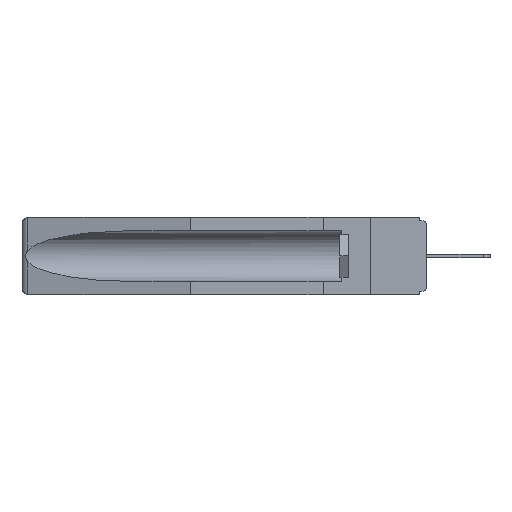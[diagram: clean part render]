
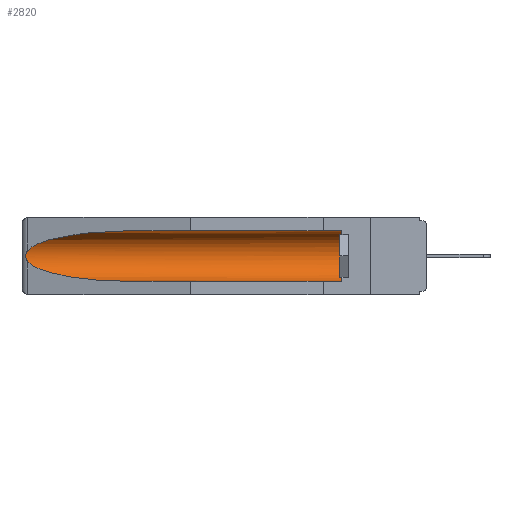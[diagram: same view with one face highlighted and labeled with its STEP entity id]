
A CAD part, left-side view. The second image highlights one B-rep face of the part: STEP entity #2820.
In plain terms, the highlighted cylindrical face has radius 2.857 mm (diameter 5.715 mm), a partial arc.
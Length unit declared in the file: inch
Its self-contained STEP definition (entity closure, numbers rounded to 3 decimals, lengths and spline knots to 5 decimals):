
#394 = VECTOR ( 'NONE', #4092, 39.37008 ) ;
#422 = EDGE_CURVE ( 'NONE', #11254, #11339, #4808, .T. ) ;
#930 = LINE ( 'NONE', #2352, #394 ) ;
#1108 = DIRECTION ( 'NONE',  ( 0., -1., 0. ) ) ;
#1222 = CARTESIAN_POINT ( 'NONE',  ( 0.26654, 1.53092, -0.15636 ) ) ;
#2047 = CARTESIAN_POINT ( 'NONE',  ( 0.155, 1.07973, -0.059 ) ) ;
#2258 = DIRECTION ( 'NONE',  ( 0., 1., 0. ) ) ;
#2352 = CARTESIAN_POINT ( 'NONE',  ( 0.155, -0.30754, -0.284 ) ) ;
#2424 = CARTESIAN_POINT ( 'NONE',  ( 0.155, -0.30754, -0.059 ) ) ;
#2436 = CARTESIAN_POINT ( 'NONE',  ( 0.155, 1.07973, -0.284 ) ) ;
#2820 = ADVANCED_FACE ( 'NONE', ( #14255 ), #13746, .F. ) ;
#2947 = CARTESIAN_POINT ( 'NONE',  ( 0.2675, 1.53308, -0.16763 ) ) ;
#3113 = CARTESIAN_POINT ( 'NONE',  ( 0.155, 1.07973, -0.059 ) ) ;
#3420 = CARTESIAN_POINT ( 'NONE',  ( 0.25451, 1.48313, -0.24835 ) ) ;
#3496 = CARTESIAN_POINT ( 'NONE',  ( 0.155, 1.07973, -0.284 ) ) ;
#3936 = AXIS2_PLACEMENT_3D ( 'NONE', #11329, #1108, #13002 ) ;
#4009 = ORIENTED_EDGE ( 'NONE', *, *, #20842, .T. ) ;
#4092 = DIRECTION ( 'NONE',  ( 0., 1., 0. ) ) ;
#4659 = CARTESIAN_POINT ( 'NONE',  ( 0.2673, 1.53269, -0.17917 ) ) ;
#4808 = LINE ( 'NONE', #2424, #13302 ) ;
#6297 = CARTESIAN_POINT ( 'NONE',  ( 0.26537, 1.52718, -0.14972 ) ) ;
#6304 = ORIENTED_EDGE ( 'NONE', *, *, #8364, .T. ) ;
#6366 = CARTESIAN_POINT ( 'NONE',  ( 0.26597, 1.5296, -0.19026 ) ) ;
#7630 = DIRECTION ( 'NONE',  ( 0., 0., 1. ) ) ;
#8026 = CARTESIAN_POINT ( 'NONE',  ( 0.26597, 1.52961, -0.15275 ) ) ;
#8206 = CIRCLE ( 'NONE', #3936, 0.1125 ) ;
#8339 = CARTESIAN_POINT ( 'NONE',  ( 0.26537, 1.52718, -0.14972 ) ) ;
#8364 = EDGE_CURVE ( 'NONE', #21430, #11004, #10285, .T. ) ;
#8382 = EDGE_LOOP ( 'NONE', ( #4009, #17523, #6304, #10797, #21688, #10684 ) ) ;
#8555 = CARTESIAN_POINT ( 'NONE',  ( 0.21114, 1.30732, -0.284 ) ) ;
#8626 = B_SPLINE_CURVE_WITH_KNOTS ( 'NONE', 3,
 ( #14704, #8026, #1222, #13124, #2947, #14777, #4659, #16411, #6366, #18053 ),
 .UNSPECIFIED., .F., .F.,
 ( 4, 2, 2, 2, 4 ),
 ( 0., 0.00029, 0.00058, 0.00087, 0.00117 ),
 .UNSPECIFIED. ) ;
#9270 = EDGE_CURVE ( 'NONE', #12674, #11254, #8206, .T. ) ;
#9860 = CARTESIAN_POINT ( 'NONE',  ( 0.155, -0.30754, -0.1715 ) ) ;
#10285 =( BOUNDED_CURVE ( )  B_SPLINE_CURVE ( 3, ( #13629, #3420, #8555, #3496 ),
 .UNSPECIFIED., .F., .F. ) 
 B_SPLINE_CURVE_WITH_KNOTS ( ( 4, 4 ),
 ( 0.1948, 1.5708 ),
 .UNSPECIFIED. ) 
 CURVE ( )  GEOMETRIC_REPRESENTATION_ITEM ( )  RATIONAL_B_SPLINE_CURVE ( ( 1., 0.848, 0.848, 1. ) ) 
 REPRESENTATION_ITEM ( '' )  );
#10684 = ORIENTED_EDGE ( 'NONE', *, *, #422, .T. ) ;
#10797 = ORIENTED_EDGE ( 'NONE', *, *, #13595, .F. ) ;
#11004 = VERTEX_POINT ( 'NONE', #2436 ) ;
#11254 = VERTEX_POINT ( 'NONE', #15301 ) ;
#11329 = CARTESIAN_POINT ( 'NONE',  ( 0.155, 0.126, -0.1715 ) ) ;
#11339 = VERTEX_POINT ( 'NONE', #2047 ) ;
#11672 = CARTESIAN_POINT ( 'NONE',  ( 0.21114, 1.30732, -0.059 ) ) ;
#12555 = CARTESIAN_POINT ( 'NONE',  ( 0.26537, 1.52718, -0.19328 ) ) ;
#12674 = VERTEX_POINT ( 'NONE', #21525 ) ;
#13002 = DIRECTION ( 'NONE',  ( 0., 0., 1. ) ) ;
#13124 = CARTESIAN_POINT ( 'NONE',  ( 0.2673, 1.5327, -0.16383 ) ) ;
#13302 = VECTOR ( 'NONE', #2258, 39.37008 ) ;
#13472 =( BOUNDED_CURVE ( )  B_SPLINE_CURVE ( 3, ( #3113, #11672, #18277, #8339 ),
 .UNSPECIFIED., .F., .F. ) 
 B_SPLINE_CURVE_WITH_KNOTS ( ( 4, 4 ),
 ( 4.71239, 6.08839 ),
 .UNSPECIFIED. ) 
 CURVE ( )  GEOMETRIC_REPRESENTATION_ITEM ( )  RATIONAL_B_SPLINE_CURVE ( ( 1., 0.848, 0.848, 1. ) ) 
 REPRESENTATION_ITEM ( '' )  );
#13595 = EDGE_CURVE ( 'NONE', #12674, #11004, #930, .T. ) ;
#13629 = CARTESIAN_POINT ( 'NONE',  ( 0.26537, 1.52718, -0.19328 ) ) ;
#13746 = CYLINDRICAL_SURFACE ( 'NONE', #18819, 0.1125 ) ;
#14255 = FACE_OUTER_BOUND ( 'NONE', #8382, .T. ) ;
#14704 = CARTESIAN_POINT ( 'NONE',  ( 0.26537, 1.52718, -0.14972 ) ) ;
#14777 = CARTESIAN_POINT ( 'NONE',  ( 0.2675, 1.53308, -0.17534 ) ) ;
#15301 = CARTESIAN_POINT ( 'NONE',  ( 0.155, 0.126, -0.059 ) ) ;
#16411 = CARTESIAN_POINT ( 'NONE',  ( 0.26655, 1.53094, -0.18657 ) ) ;
#17060 = DIRECTION ( 'NONE',  ( 0., 1., 0. ) ) ;
#17523 = ORIENTED_EDGE ( 'NONE', *, *, #17722, .T. ) ;
#17712 = VERTEX_POINT ( 'NONE', #6297 ) ;
#17722 = EDGE_CURVE ( 'NONE', #17712, #21430, #8626, .T. ) ;
#18053 = CARTESIAN_POINT ( 'NONE',  ( 0.26537, 1.52718, -0.19328 ) ) ;
#18277 = CARTESIAN_POINT ( 'NONE',  ( 0.25451, 1.48313, -0.09465 ) ) ;
#18819 = AXIS2_PLACEMENT_3D ( 'NONE', #9860, #17060, #7630 ) ;
#20842 = EDGE_CURVE ( 'NONE', #11339, #17712, #13472, .T. ) ;
#21430 = VERTEX_POINT ( 'NONE', #12555 ) ;
#21525 = CARTESIAN_POINT ( 'NONE',  ( 0.155, 0.126, -0.284 ) ) ;
#21688 = ORIENTED_EDGE ( 'NONE', *, *, #9270, .T. ) ;
